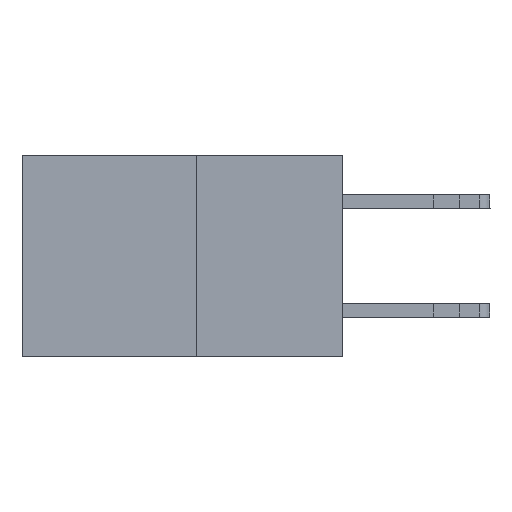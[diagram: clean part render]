
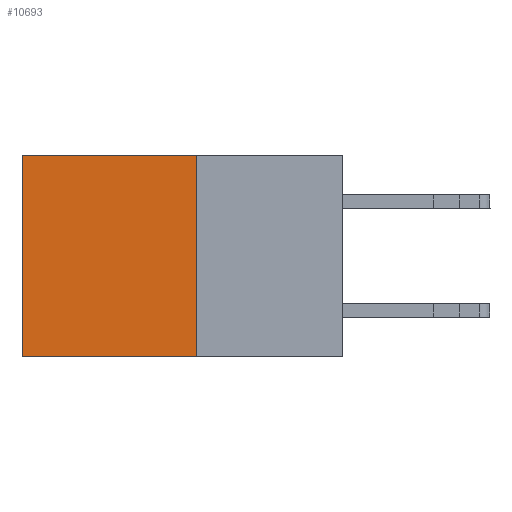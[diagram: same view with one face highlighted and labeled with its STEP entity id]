
A CAD part, left-side view. The second image highlights one B-rep face of the part: STEP entity #10693.
In plain terms, the highlighted planar face has unit normal (-1, 0, 0).
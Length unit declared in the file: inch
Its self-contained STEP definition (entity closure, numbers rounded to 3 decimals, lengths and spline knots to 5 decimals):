
#83 = CARTESIAN_POINT ( 'NONE',  ( 0.277, 0.59, -0.37 ) ) ;
#1758 = EDGE_CURVE ( 'NONE', #7841, #17086, #17419, .T. ) ;
#2404 = LINE ( 'NONE', #7435, #6662 ) ;
#4125 = EDGE_CURVE ( 'NONE', #16400, #17086, #11098, .T. ) ;
#4246 = CARTESIAN_POINT ( 'NONE',  ( 0.277, 0.59, 0. ) ) ;
#4607 = VECTOR ( 'NONE', #17098, 39.37008 ) ;
#5291 = ORIENTED_EDGE ( 'NONE', *, *, #4125, .F. ) ;
#6021 = CARTESIAN_POINT ( 'NONE',  ( 0.277, 0.59, -0.37 ) ) ;
#6059 = DIRECTION ( 'NONE',  ( 0., 0., -1. ) ) ;
#6062 = DIRECTION ( 'NONE',  ( 1., 0., 0. ) ) ;
#6126 = CARTESIAN_POINT ( 'NONE',  ( 0.277, 0.27, -0.37 ) ) ;
#6160 = PLANE ( 'NONE',  #9485 ) ;
#6384 = DIRECTION ( 'NONE',  ( 0., 0., -1. ) ) ;
#6662 = VECTOR ( 'NONE', #7378, 39.37008 ) ;
#7378 = DIRECTION ( 'NONE',  ( 0., 1., 0. ) ) ;
#7435 = CARTESIAN_POINT ( 'NONE',  ( 0.277, 0.27, 0. ) ) ;
#7726 = VECTOR ( 'NONE', #6384, 39.37008 ) ;
#7841 = VERTEX_POINT ( 'NONE', #4246 ) ;
#8378 = CARTESIAN_POINT ( 'NONE',  ( 0.277, 0.27, -0.37 ) ) ;
#8798 = CARTESIAN_POINT ( 'NONE',  ( 0.277, 0.27, -0.37 ) ) ;
#9188 = ORIENTED_EDGE ( 'NONE', *, *, #1758, .T. ) ;
#9485 = AXIS2_PLACEMENT_3D ( 'NONE', #6126, #6062, #6059 ) ;
#10323 = LINE ( 'NONE', #13855, #17621 ) ;
#10472 = ORIENTED_EDGE ( 'NONE', *, *, #11533, .F. ) ;
#10536 = EDGE_CURVE ( 'NONE', #17353, #7841, #2404, .T. ) ;
#10693 = ADVANCED_FACE ( 'NONE', ( #17401 ), #6160, .F. ) ;
#11098 = LINE ( 'NONE', #8378, #4607 ) ;
#11533 = EDGE_CURVE ( 'NONE', #17353, #16400, #10323, .T. ) ;
#13811 = DIRECTION ( 'NONE',  ( 0., 0., -1. ) ) ;
#13855 = CARTESIAN_POINT ( 'NONE',  ( 0.277, 0.27, -0.37 ) ) ;
#13986 = EDGE_LOOP ( 'NONE', ( #9188, #5291, #10472, #14106 ) ) ;
#14106 = ORIENTED_EDGE ( 'NONE', *, *, #10536, .T. ) ;
#14857 = CARTESIAN_POINT ( 'NONE',  ( 0.277, 0.27, 0. ) ) ;
#16400 = VERTEX_POINT ( 'NONE', #8798 ) ;
#17086 = VERTEX_POINT ( 'NONE', #83 ) ;
#17098 = DIRECTION ( 'NONE',  ( 0., 1., 0. ) ) ;
#17353 = VERTEX_POINT ( 'NONE', #14857 ) ;
#17401 = FACE_OUTER_BOUND ( 'NONE', #13986, .T. ) ;
#17419 = LINE ( 'NONE', #6021, #7726 ) ;
#17621 = VECTOR ( 'NONE', #13811, 39.37008 ) ;
